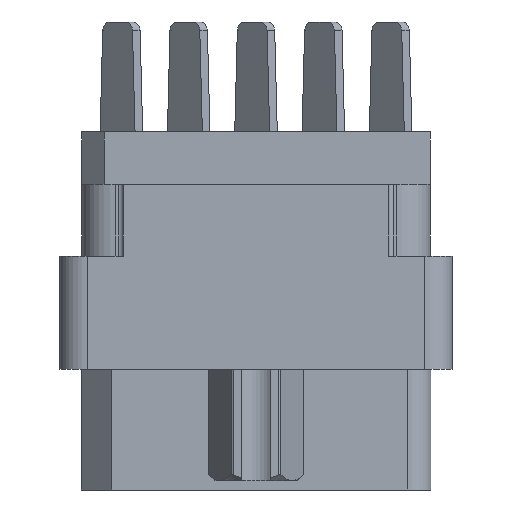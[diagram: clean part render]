
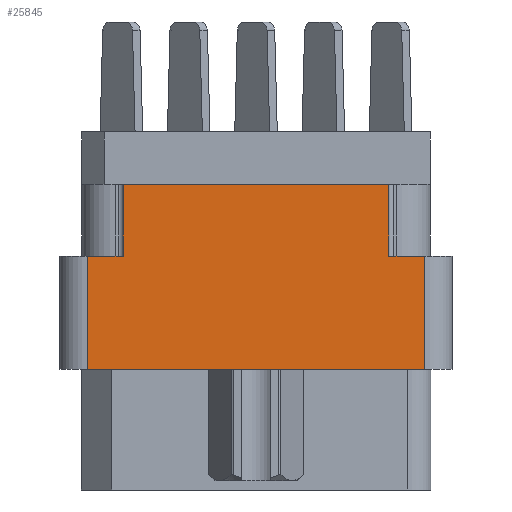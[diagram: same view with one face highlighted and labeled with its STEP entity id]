
A CAD part, left-side view. The second image highlights one B-rep face of the part: STEP entity #25845.
In plain terms, the highlighted planar face has unit normal (-1, 0, 0).
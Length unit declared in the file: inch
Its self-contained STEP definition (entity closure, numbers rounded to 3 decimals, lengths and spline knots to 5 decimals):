
#1466 = CARTESIAN_POINT ( 'NONE',  ( -1., -0.376, -0.529 ) ) ;
#2830 = PLANE ( 'NONE',  #36474 ) ;
#3362 = LINE ( 'NONE', #41657, #44804 ) ;
#4703 = DIRECTION ( 'NONE',  ( 0., 0., 1. ) ) ;
#5726 = CARTESIAN_POINT ( 'NONE',  ( -1., -0.376, -0.798 ) ) ;
#5950 = DIRECTION ( 'NONE',  ( 0., 0., 1. ) ) ;
#7562 = LINE ( 'NONE', #31714, #32639 ) ;
#8429 = LINE ( 'NONE', #11847, #31173 ) ;
#8829 = CARTESIAN_POINT ( 'NONE',  ( -1., -0.296, -0.277 ) ) ;
#9291 = ORIENTED_EDGE ( 'NONE', *, *, #15610, .F. ) ;
#9340 = CARTESIAN_POINT ( 'NONE',  ( -1., 0.438, -0.117 ) ) ;
#10019 = DIRECTION ( 'NONE',  ( 0., -1., 0. ) ) ;
#10636 = LINE ( 'NONE', #20899, #43972 ) ;
#11420 = ORIENTED_EDGE ( 'NONE', *, *, #33794, .F. ) ;
#11847 = CARTESIAN_POINT ( 'NONE',  ( -1., 0.296, -0.277 ) ) ;
#13906 = CARTESIAN_POINT ( 'NONE',  ( -1., -0.296, -0.277 ) ) ;
#15101 = EDGE_CURVE ( 'NONE', #22770, #19578, #7562, .T. ) ;
#15610 = EDGE_CURVE ( 'NONE', #19578, #20971, #39579, .T. ) ;
#16129 = DIRECTION ( 'NONE',  ( 0., -1., 0. ) ) ;
#16506 = VECTOR ( 'NONE', #10019, 39.37008 ) ;
#16973 = CARTESIAN_POINT ( 'NONE',  ( -1., -0.376, -0.798 ) ) ;
#17194 = DIRECTION ( 'NONE',  ( 0., 0., 1. ) ) ;
#17209 = VERTEX_POINT ( 'NONE', #41123 ) ;
#17955 = EDGE_CURVE ( 'NONE', #21921, #30811, #44157, .T. ) ;
#18178 = CARTESIAN_POINT ( 'NONE',  ( -1., 0.376, -0.798 ) ) ;
#18495 = EDGE_LOOP ( 'NONE', ( #9291, #36045, #27796, #43952, #34774, #22223, #11420, #40410 ) ) ;
#19578 = VERTEX_POINT ( 'NONE', #29598 ) ;
#20394 = FACE_OUTER_BOUND ( 'NONE', #18495, .T. ) ;
#20465 = EDGE_CURVE ( 'NONE', #20971, #34481, #3362, .T. ) ;
#20899 = CARTESIAN_POINT ( 'NONE',  ( -1., -0.296, -0.277 ) ) ;
#20971 = VERTEX_POINT ( 'NONE', #21313 ) ;
#21313 = CARTESIAN_POINT ( 'NONE',  ( -1., 0.376, -0.277 ) ) ;
#21746 = EDGE_CURVE ( 'NONE', #22770, #30811, #36516, .T. ) ;
#21921 = VERTEX_POINT ( 'NONE', #13906 ) ;
#22223 = ORIENTED_EDGE ( 'NONE', *, *, #32020, .F. ) ;
#22770 = VERTEX_POINT ( 'NONE', #1466 ) ;
#25845 = ADVANCED_FACE ( 'NONE', ( #20394 ), #2830, .T. ) ;
#27796 = ORIENTED_EDGE ( 'NONE', *, *, #21746, .T. ) ;
#28329 = CARTESIAN_POINT ( 'NONE',  ( -1., 0.296, -0.117 ) ) ;
#29015 = VECTOR ( 'NONE', #4703, 39.37008 ) ;
#29598 = CARTESIAN_POINT ( 'NONE',  ( -1., 0.376, -0.529 ) ) ;
#30811 = VERTEX_POINT ( 'NONE', #42961 ) ;
#31173 = VECTOR ( 'NONE', #43753, 39.37008 ) ;
#31393 = DIRECTION ( 'NONE',  ( 0., -1., 0. ) ) ;
#31714 = CARTESIAN_POINT ( 'NONE',  ( -1., -0.376, -0.529 ) ) ;
#32020 = EDGE_CURVE ( 'NONE', #41359, #17209, #44660, .T. ) ;
#32639 = VECTOR ( 'NONE', #38787, 39.37008 ) ;
#33784 = VECTOR ( 'NONE', #16129, 39.37008 ) ;
#33794 = EDGE_CURVE ( 'NONE', #34481, #41359, #8429, .T. ) ;
#34481 = VERTEX_POINT ( 'NONE', #41410 ) ;
#34512 = DIRECTION ( 'NONE',  ( -1., 0., 0. ) ) ;
#34774 = ORIENTED_EDGE ( 'NONE', *, *, #39194, .T. ) ;
#36045 = ORIENTED_EDGE ( 'NONE', *, *, #15101, .F. ) ;
#36474 = AXIS2_PLACEMENT_3D ( 'NONE', #16973, #34512, #17194 ) ;
#36516 = LINE ( 'NONE', #5726, #41167 ) ;
#38787 = DIRECTION ( 'NONE',  ( 0., 1., 0. ) ) ;
#39194 = EDGE_CURVE ( 'NONE', #21921, #17209, #10636, .T. ) ;
#39579 = LINE ( 'NONE', #18178, #29015 ) ;
#40410 = ORIENTED_EDGE ( 'NONE', *, *, #20465, .F. ) ;
#41123 = CARTESIAN_POINT ( 'NONE',  ( -1., -0.296, -0.117 ) ) ;
#41167 = VECTOR ( 'NONE', #5950, 39.37008 ) ;
#41359 = VERTEX_POINT ( 'NONE', #28329 ) ;
#41410 = CARTESIAN_POINT ( 'NONE',  ( -1., 0.296, -0.277 ) ) ;
#41657 = CARTESIAN_POINT ( 'NONE',  ( -1., 0.438, -0.277 ) ) ;
#42961 = CARTESIAN_POINT ( 'NONE',  ( -1., -0.376, -0.277 ) ) ;
#43753 = DIRECTION ( 'NONE',  ( 0., 0., 1. ) ) ;
#43952 = ORIENTED_EDGE ( 'NONE', *, *, #17955, .F. ) ;
#43972 = VECTOR ( 'NONE', #44822, 39.37008 ) ;
#44157 = LINE ( 'NONE', #8829, #33784 ) ;
#44660 = LINE ( 'NONE', #9340, #16506 ) ;
#44804 = VECTOR ( 'NONE', #31393, 39.37008 ) ;
#44822 = DIRECTION ( 'NONE',  ( 0., 0., 1. ) ) ;
